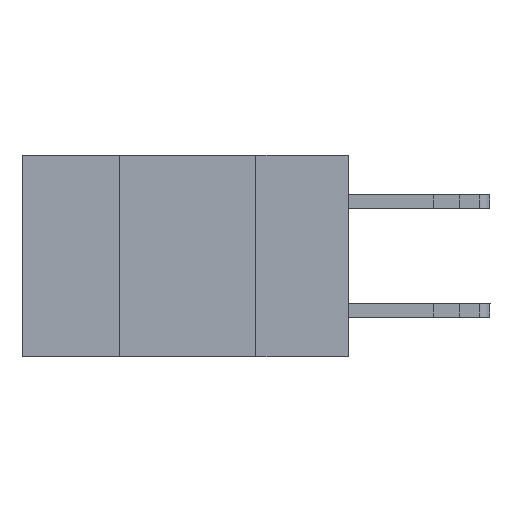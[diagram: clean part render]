
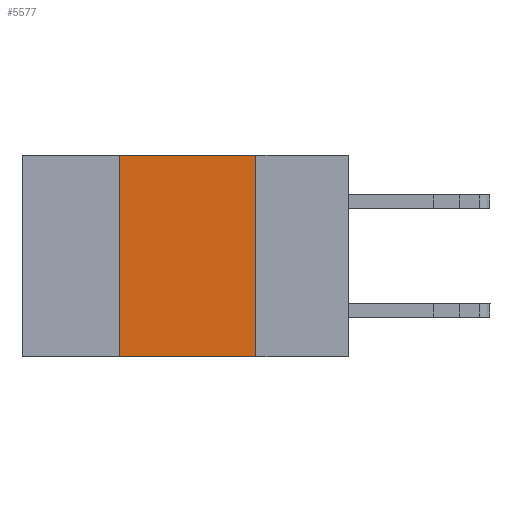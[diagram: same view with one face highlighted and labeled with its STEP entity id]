
A CAD part, left-side view. The second image highlights one B-rep face of the part: STEP entity #5577.
In plain terms, the highlighted planar face has unit normal (-1, 0, 0).
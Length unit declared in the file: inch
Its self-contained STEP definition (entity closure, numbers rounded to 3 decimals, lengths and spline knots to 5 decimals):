
#221 = LINE ( 'NONE', #2156, #15465 ) ;
#1865 = DIRECTION ( 'NONE',  ( 0., -1., 0. ) ) ;
#2156 = CARTESIAN_POINT ( 'NONE',  ( 0., 0.6, -0.37 ) ) ;
#4218 = CARTESIAN_POINT ( 'NONE',  ( 0., 0.17, -0.37 ) ) ;
#4842 = VERTEX_POINT ( 'NONE', #18117 ) ;
#5130 = DIRECTION ( 'NONE',  ( 0., 0., 1. ) ) ;
#5156 = CARTESIAN_POINT ( 'NONE',  ( 0., 0.42, -0.37 ) ) ;
#5221 = EDGE_CURVE ( 'NONE', #14743, #4842, #16562, .T. ) ;
#5317 = EDGE_CURVE ( 'NONE', #14743, #9370, #221, .T. ) ;
#5443 = FACE_OUTER_BOUND ( 'NONE', #16192, .T. ) ;
#5577 = ADVANCED_FACE ( 'NONE', ( #5443 ), #11911, .F. ) ;
#5976 = ORIENTED_EDGE ( 'NONE', *, *, #6131, .F. ) ;
#6131 = EDGE_CURVE ( 'NONE', #4842, #11449, #13479, .T. ) ;
#6153 = CARTESIAN_POINT ( 'NONE',  ( 0., 0.17, 0. ) ) ;
#6212 = VECTOR ( 'NONE', #5130, 39.37008 ) ;
#6375 = EDGE_CURVE ( 'NONE', #11449, #9370, #10622, .T. ) ;
#7350 = VECTOR ( 'NONE', #13494, 39.37008 ) ;
#8574 = CARTESIAN_POINT ( 'NONE',  ( 0., 0.42, -0.37 ) ) ;
#9370 = VERTEX_POINT ( 'NONE', #4218 ) ;
#9748 = VECTOR ( 'NONE', #16176, 39.37008 ) ;
#10622 = LINE ( 'NONE', #13506, #7350 ) ;
#11164 = ORIENTED_EDGE ( 'NONE', *, *, #5221, .F. ) ;
#11449 = VERTEX_POINT ( 'NONE', #6153 ) ;
#11588 = ORIENTED_EDGE ( 'NONE', *, *, #5317, .T. ) ;
#11860 = DIRECTION ( 'NONE',  ( 0., 0., -1. ) ) ;
#11890 = DIRECTION ( 'NONE',  ( 1., 0., 0. ) ) ;
#11911 = PLANE ( 'NONE',  #18555 ) ;
#12220 = ORIENTED_EDGE ( 'NONE', *, *, #6375, .F. ) ;
#12904 = CARTESIAN_POINT ( 'NONE',  ( 0., 0.6, 0. ) ) ;
#13479 = LINE ( 'NONE', #16348, #9748 ) ;
#13494 = DIRECTION ( 'NONE',  ( 0., 0., -1. ) ) ;
#13506 = CARTESIAN_POINT ( 'NONE',  ( 0., 0.17, -0.37 ) ) ;
#14743 = VERTEX_POINT ( 'NONE', #8574 ) ;
#15465 = VECTOR ( 'NONE', #1865, 39.37008 ) ;
#16176 = DIRECTION ( 'NONE',  ( 0., -1., 0. ) ) ;
#16192 = EDGE_LOOP ( 'NONE', ( #12220, #5976, #11164, #11588 ) ) ;
#16348 = CARTESIAN_POINT ( 'NONE',  ( 0., 0.6, 0. ) ) ;
#16562 = LINE ( 'NONE', #5156, #6212 ) ;
#18117 = CARTESIAN_POINT ( 'NONE',  ( 0., 0.42, 0. ) ) ;
#18555 = AXIS2_PLACEMENT_3D ( 'NONE', #12904, #11890, #11860 ) ;
